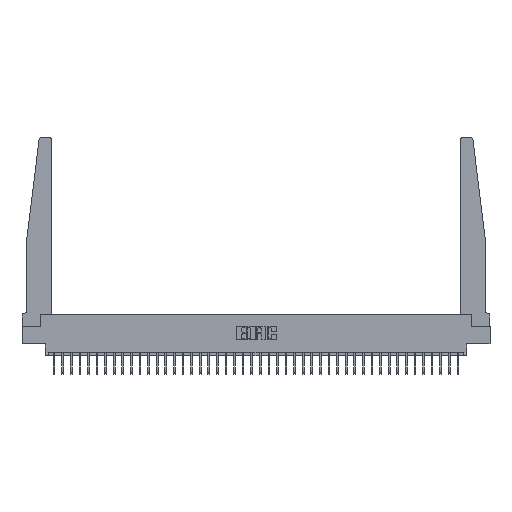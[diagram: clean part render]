
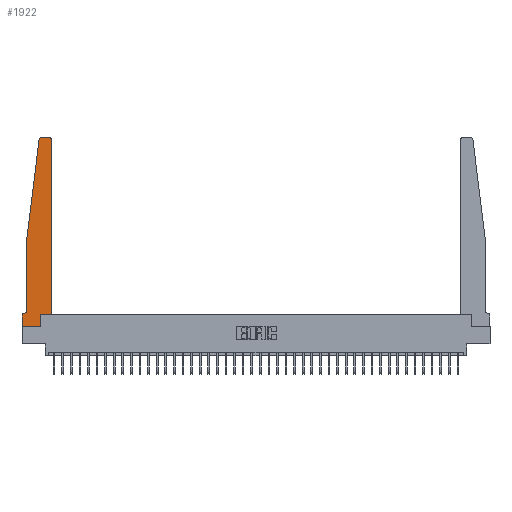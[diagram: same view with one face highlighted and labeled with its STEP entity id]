
A CAD part, top view. The second image highlights one B-rep face of the part: STEP entity #1922.
In plain terms, the highlighted planar face has unit normal (0, 0, 1).
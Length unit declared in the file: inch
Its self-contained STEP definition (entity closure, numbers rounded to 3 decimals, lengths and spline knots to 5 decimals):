
#930 = VECTOR ( 'NONE', #25880, 39.37008 ) ;
#1453 = FACE_OUTER_BOUND ( 'NONE', #3373, .T. ) ;
#1468 = LINE ( 'NONE', #29231, #14543 ) ;
#1625 = EDGE_CURVE ( 'NONE', #37048, #7731, #16813, .T. ) ;
#1922 = ADVANCED_FACE ( 'NONE', ( #1453 ), #13294, .T. ) ;
#2058 = VERTEX_POINT ( 'NONE', #24782 ) ;
#2933 = CARTESIAN_POINT ( 'NONE',  ( 0., 0.1875, 0.37 ) ) ;
#3227 = DIRECTION ( 'NONE',  ( 0., 1., 0. ) ) ;
#3373 = EDGE_LOOP ( 'NONE', ( #32935, #14502, #11572, #12953, #11887, #4706, #22349, #8825, #18811, #5907, #28101, #27657 ) ) ;
#3429 = DIRECTION ( 'NONE',  ( -1., 0., 0. ) ) ;
#3682 = DIRECTION ( 'NONE',  ( -1., 0., 0. ) ) ;
#4392 = CARTESIAN_POINT ( 'NONE',  ( 0.24675, 2.72367, 0.37 ) ) ;
#4660 = CARTESIAN_POINT ( 'NONE',  ( 0.395, 2.75, 0.37 ) ) ;
#4706 = ORIENTED_EDGE ( 'NONE', *, *, #11645, .T. ) ;
#5684 = EDGE_CURVE ( 'NONE', #14397, #37048, #32108, .T. ) ;
#5709 = EDGE_CURVE ( 'NONE', #33837, #14397, #1468, .T. ) ;
#5857 = LINE ( 'NONE', #33874, #15334 ) ;
#5907 = ORIENTED_EDGE ( 'NONE', *, *, #22399, .T. ) ;
#6125 = CARTESIAN_POINT ( 'NONE',  ( 0.425, 0.18, 0.37 ) ) ;
#6233 = CARTESIAN_POINT ( 'NONE',  ( 0.425, 0.18, 0.37 ) ) ;
#6700 = EDGE_CURVE ( 'NONE', #34190, #12920, #7716, .T. ) ;
#7233 = EDGE_CURVE ( 'NONE', #26559, #13473, #5857, .T. ) ;
#7459 = EDGE_CURVE ( 'NONE', #16788, #26559, #11229, .T. ) ;
#7524 = LINE ( 'NONE', #6233, #34518 ) ;
#7716 = LINE ( 'NONE', #8760, #930 ) ;
#7731 = VERTEX_POINT ( 'NONE', #15748 ) ;
#8760 = CARTESIAN_POINT ( 'NONE',  ( 0.425, 0.18, 0.37 ) ) ;
#8825 = ORIENTED_EDGE ( 'NONE', *, *, #7459, .T. ) ;
#10027 = DIRECTION ( 'NONE',  ( 0., 0., 1. ) ) ;
#10057 = DIRECTION ( 'NONE',  ( 1., 0., 0. ) ) ;
#10323 = DIRECTION ( 'NONE',  ( 0., -1., 0. ) ) ;
#10490 = CARTESIAN_POINT ( 'NONE',  ( 0.065, 0.2375, 0.37 ) ) ;
#10860 = CIRCLE ( 'NONE', #30810, 0.03 ) ;
#11229 = LINE ( 'NONE', #11827, #31502 ) ;
#11306 = CIRCLE ( 'NONE', #18364, 0.03 ) ;
#11572 = ORIENTED_EDGE ( 'NONE', *, *, #5709, .T. ) ;
#11645 = EDGE_CURVE ( 'NONE', #7731, #28149, #31696, .T. ) ;
#11701 = DIRECTION ( 'NONE',  ( 1., 0., 0. ) ) ;
#11827 = CARTESIAN_POINT ( 'NONE',  ( 0., 0., 0.37 ) ) ;
#11861 = DIRECTION ( 'NONE',  ( -1., 0., 0. ) ) ;
#11887 = ORIENTED_EDGE ( 'NONE', *, *, #1625, .T. ) ;
#11977 = DIRECTION ( 'NONE',  ( -0.122, -0.992, 0. ) ) ;
#11990 = DIRECTION ( 'NONE',  ( 1., 0., 0. ) ) ;
#12177 = CARTESIAN_POINT ( 'NONE',  ( 0., 0., 0.37 ) ) ;
#12479 = CARTESIAN_POINT ( 'NONE',  ( 0.425, 2.72, 0.37 ) ) ;
#12500 = VECTOR ( 'NONE', #3682, 39.37008 ) ;
#12920 = VERTEX_POINT ( 'NONE', #12479 ) ;
#12953 = ORIENTED_EDGE ( 'NONE', *, *, #5684, .T. ) ;
#13160 = DIRECTION ( 'NONE',  ( 1., 0., 0. ) ) ;
#13294 = PLANE ( 'NONE',  #34362 ) ;
#13473 = VERTEX_POINT ( 'NONE', #16482 ) ;
#14397 = VERTEX_POINT ( 'NONE', #26355 ) ;
#14502 = ORIENTED_EDGE ( 'NONE', *, *, #33859, .T. ) ;
#14543 = VECTOR ( 'NONE', #11977, 39.37008 ) ;
#14575 = AXIS2_PLACEMENT_3D ( 'NONE', #17886, #31897, #3429 ) ;
#15110 = DIRECTION ( 'NONE',  ( 0., -1., 0. ) ) ;
#15334 = VECTOR ( 'NONE', #3227, 39.37008 ) ;
#15748 = CARTESIAN_POINT ( 'NONE',  ( 0.015, 0.1875, 0.37 ) ) ;
#16482 = CARTESIAN_POINT ( 'NONE',  ( 0.2605, 0.18, 0.37 ) ) ;
#16788 = VERTEX_POINT ( 'NONE', #36834 ) ;
#16813 = CIRCLE ( 'NONE', #14575, 0.05 ) ;
#16972 = EDGE_CURVE ( 'NONE', #23162, #2058, #26050, .T. ) ;
#17149 = CARTESIAN_POINT ( 'NONE',  ( 0.065, 0.1875, 0.37 ) ) ;
#17886 = CARTESIAN_POINT ( 'NONE',  ( 0.015, 0.2375, 0.37 ) ) ;
#18364 = AXIS2_PLACEMENT_3D ( 'NONE', #29345, #35630, #10057 ) ;
#18383 = CARTESIAN_POINT ( 'NONE',  ( 0.25, 2.75, 0.37 ) ) ;
#18586 = CARTESIAN_POINT ( 'NONE',  ( 0.2605, 0., 0.37 ) ) ;
#18715 = EDGE_CURVE ( 'NONE', #12920, #23162, #11306, .T. ) ;
#18811 = ORIENTED_EDGE ( 'NONE', *, *, #7233, .T. ) ;
#20223 = LINE ( 'NONE', #12177, #31938 ) ;
#22231 = VECTOR ( 'NONE', #11861, 39.37008 ) ;
#22349 = ORIENTED_EDGE ( 'NONE', *, *, #35507, .T. ) ;
#22399 = EDGE_CURVE ( 'NONE', #13473, #34190, #7524, .T. ) ;
#23162 = VERTEX_POINT ( 'NONE', #4660 ) ;
#24782 = CARTESIAN_POINT ( 'NONE',  ( 0.27653, 2.75, 0.37 ) ) ;
#25880 = DIRECTION ( 'NONE',  ( 0., 1., 0. ) ) ;
#26050 = LINE ( 'NONE', #18383, #12500 ) ;
#26355 = CARTESIAN_POINT ( 'NONE',  ( 0.065, 1.25, 0.37 ) ) ;
#26559 = VERTEX_POINT ( 'NONE', #18586 ) ;
#27657 = ORIENTED_EDGE ( 'NONE', *, *, #18715, .T. ) ;
#28101 = ORIENTED_EDGE ( 'NONE', *, *, #6700, .T. ) ;
#28149 = VERTEX_POINT ( 'NONE', #2933 ) ;
#29231 = CARTESIAN_POINT ( 'NONE',  ( 0.065, 1.25, 0.37 ) ) ;
#29345 = CARTESIAN_POINT ( 'NONE',  ( 0.395, 2.72, 0.37 ) ) ;
#29492 = CARTESIAN_POINT ( 'NONE',  ( 0.065, 1.25, 0.37 ) ) ;
#30068 = CARTESIAN_POINT ( 'NONE',  ( 0.27653, 2.72, 0.37 ) ) ;
#30418 = DIRECTION ( 'NONE',  ( 0., 0., 1. ) ) ;
#30810 = AXIS2_PLACEMENT_3D ( 'NONE', #30068, #10027, #33203 ) ;
#31502 = VECTOR ( 'NONE', #11701, 39.37008 ) ;
#31647 = VECTOR ( 'NONE', #10323, 39.37008 ) ;
#31696 = LINE ( 'NONE', #17149, #22231 ) ;
#31897 = DIRECTION ( 'NONE',  ( 0., 0., -1. ) ) ;
#31938 = VECTOR ( 'NONE', #15110, 39.37008 ) ;
#32108 = LINE ( 'NONE', #29492, #31647 ) ;
#32935 = ORIENTED_EDGE ( 'NONE', *, *, #16972, .T. ) ;
#33203 = DIRECTION ( 'NONE',  ( 1., 0., 0. ) ) ;
#33837 = VERTEX_POINT ( 'NONE', #4392 ) ;
#33859 = EDGE_CURVE ( 'NONE', #2058, #33837, #10860, .T. ) ;
#33874 = CARTESIAN_POINT ( 'NONE',  ( 0.2605, 0.18, 0.37 ) ) ;
#34190 = VERTEX_POINT ( 'NONE', #6125 ) ;
#34362 = AXIS2_PLACEMENT_3D ( 'NONE', #36061, #30418, #13160 ) ;
#34518 = VECTOR ( 'NONE', #11990, 39.37008 ) ;
#35507 = EDGE_CURVE ( 'NONE', #28149, #16788, #20223, .T. ) ;
#35630 = DIRECTION ( 'NONE',  ( 0., 0., 1. ) ) ;
#36061 = CARTESIAN_POINT ( 'NONE',  ( 0., 0.1875, 0.37 ) ) ;
#36834 = CARTESIAN_POINT ( 'NONE',  ( 0., 0., 0.37 ) ) ;
#37048 = VERTEX_POINT ( 'NONE', #10490 ) ;
